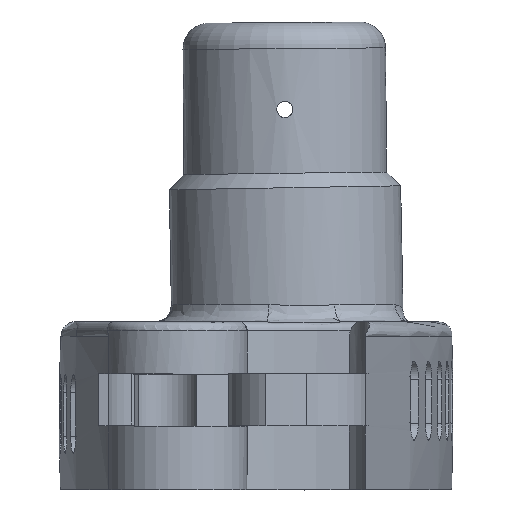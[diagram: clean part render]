
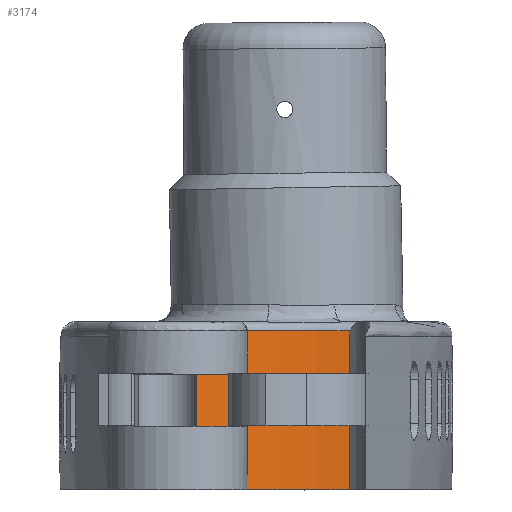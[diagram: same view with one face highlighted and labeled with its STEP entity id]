
A CAD part, front view. The second image highlights one B-rep face of the part: STEP entity #3174.
In plain terms, the highlighted cylindrical face has radius 46.197 mm (diameter 92.394 mm), a partial arc.
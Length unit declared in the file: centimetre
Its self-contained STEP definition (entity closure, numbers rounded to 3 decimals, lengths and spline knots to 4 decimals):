
#128=CIRCLE($,#3346,4.6197);
#177=CIRCLE($,#3433,4.6197);
#435=FACE_OUTER_BOUND($,#657,.T.);
#657=EDGE_LOOP($,(#2546,#2547,#2548,#2549,#2550,#2551,#2552));
#804=LINE($,#15034,#948);
#806=LINE($,#15040,#950);
#811=LINE($,#15164,#955);
#812=LINE($,#15169,#956);
#948=VECTOR($,#3922,1.1);
#950=VECTOR($,#3928,0.75);
#955=VECTOR($,#3965,2.65);
#956=VECTOR($,#3974,0.9);
#1130=B_SPLINE_CURVE_WITH_KNOTS($,3,(#5941,#5942,#5943,#5944,#5945,#5946,
#5947),.UNSPECIFIED.,.F.,.F.,(4,3,4),(0.8253,0.9054,
0.929),.UNSPECIFIED.);
#1320=VERTEX_POINT($,#5530);
#1321=VERTEX_POINT($,#5543);
#1349=VERTEX_POINT($,#5940);
#1398=VERTEX_POINT($,#15020);
#1404=VERTEX_POINT($,#15032);
#1406=VERTEX_POINT($,#15038);
#1413=VERTEX_POINT($,#15163);
#1692=EDGE_CURVE($,#1320,#1321,#128,.T.);
#1728=EDGE_CURVE($,#1321,#1349,#1130,.F.);
#1801=EDGE_CURVE($,#1398,#1404,#804,.T.);
#1804=EDGE_CURVE($,#1320,#1406,#806,.T.);
#1816=EDGE_CURVE($,#1349,#1413,#811,.T.);
#1819=EDGE_CURVE($,#1406,#1398,#812,.T.);
#1820=EDGE_CURVE($,#1413,#1404,#177,.T.);
#2546=ORIENTED_EDGE($,*,*,#1692,.F.);
#2547=ORIENTED_EDGE($,*,*,#1804,.T.);
#2548=ORIENTED_EDGE($,*,*,#1819,.T.);
#2549=ORIENTED_EDGE($,*,*,#1801,.T.);
#2550=ORIENTED_EDGE($,*,*,#1820,.F.);
#2551=ORIENTED_EDGE($,*,*,#1816,.F.);
#2552=ORIENTED_EDGE($,*,*,#1728,.F.);
#3034=CYLINDRICAL_SURFACE($,#3432,4.6197);
#3174=ADVANCED_FACE($,(#435),#3034,.F.);
#3346=AXIS2_PLACEMENT_3D($,#5544,#3783,#3784);
#3432=AXIS2_PLACEMENT_3D($,#15168,#3972,#3973);
#3433=AXIS2_PLACEMENT_3D($,#15170,#3975,#3976);
#3783=DIRECTION('center_axis',(0.,-0.001,
-1.));
#3784=DIRECTION('ref_axis',(-0.141,0.99,0.));
#3922=DIRECTION($,(0.,-0.001,-1.));
#3928=DIRECTION($,(0.,-0.001,-1.));
#3965=DIRECTION($,(0.,-0.001,-1.));
#3972=DIRECTION('center_axis',(0.,0.001,
1.));
#3973=DIRECTION('ref_axis',(0.225,0.974,-0.001));
#3974=DIRECTION($,(0.,-0.001,-1.));
#3975=DIRECTION('center_axis',(0.,0.001,
1.));
#3976=DIRECTION('ref_axis',(0.225,0.974,-0.001));
#5530=CARTESIAN_POINT('',(-16.5496,20.6559,2.7527));
#5543=CARTESIAN_POINT('',(-13.0001,21.2592,2.7521));
#5544=CARTESIAN_POINT('Origin',(-14.062,16.7631,2.7545));
#5940=CARTESIAN_POINT('',(-13.022,21.2642,2.6521));
#5941=CARTESIAN_POINT('Ctrl Pts',(-13.022,21.2642,2.6521));
#5942=CARTESIAN_POINT('Ctrl Pts',(-13.022,21.2642,2.6788));
#5943=CARTESIAN_POINT('Ctrl Pts',(-13.0175,21.2632,2.7052));
#5944=CARTESIAN_POINT('Ctrl Pts',(-13.0088,21.2612,2.7304));
#5945=CARTESIAN_POINT('Ctrl Pts',(-13.0063,21.2606,2.7378));
#5946=CARTESIAN_POINT('Ctrl Pts',(-13.0034,21.2599,2.745));
#5947=CARTESIAN_POINT('Ctrl Pts',(-13.0001,21.2592,2.7521));
#15020=CARTESIAN_POINT('',(-16.5498,20.655,1.1027));
#15032=CARTESIAN_POINT('',(-16.5498,20.6545,0.0027));
#15034=CARTESIAN_POINT($,(-16.5496,20.6559,2.9027));
#15038=CARTESIAN_POINT('',(-16.5497,20.6555,2.0027));
#15040=CARTESIAN_POINT($,(-16.5496,20.6559,2.9027));
#15163=CARTESIAN_POINT('',(-13.0222,21.2629,0.0021));
#15164=CARTESIAN_POINT($,(-13.0219,21.2644,2.9021));
#15168=CARTESIAN_POINT('Origin',(-14.0619,16.7632,2.9045));
#15169=CARTESIAN_POINT($,(-16.5497,20.6555,2.0027));
#15170=CARTESIAN_POINT('Origin',(-14.0622,16.7617,0.0045));
